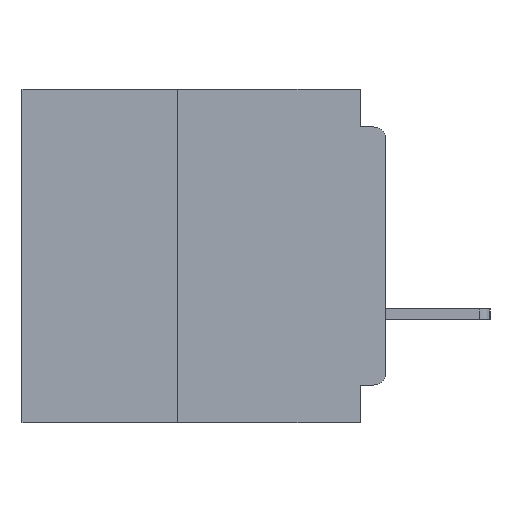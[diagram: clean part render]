
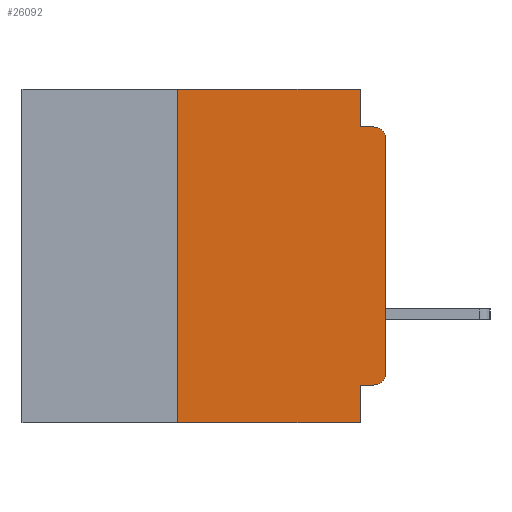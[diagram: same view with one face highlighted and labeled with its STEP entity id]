
A CAD part, left-side view. The second image highlights one B-rep face of the part: STEP entity #26092.
In plain terms, the highlighted planar face has unit normal (-1, 0, 0).
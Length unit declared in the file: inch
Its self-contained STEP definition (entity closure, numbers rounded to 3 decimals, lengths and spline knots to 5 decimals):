
#500 = CARTESIAN_POINT ( 'NONE',  ( 0., 0.437, 0. ) ) ;
#992 = VERTEX_POINT ( 'NONE', #31746 ) ;
#1232 = EDGE_CURVE ( 'NONE', #992, #51949, #61329, .T. ) ;
#2857 = CARTESIAN_POINT ( 'NONE',  ( 0., 0.031, 0. ) ) ;
#4072 = CARTESIAN_POINT ( 'NONE',  ( 0., 0.031, -0.045 ) ) ;
#5581 = VERTEX_POINT ( 'NONE', #11005 ) ;
#5593 = DIRECTION ( 'NONE',  ( 0., 0., 1. ) ) ;
#6571 = DIRECTION ( 'NONE',  ( 0., 1., 0. ) ) ;
#6765 = CARTESIAN_POINT ( 'NONE',  ( 0., 0., -0.045 ) ) ;
#6943 = AXIS2_PLACEMENT_3D ( 'NONE', #26610, #61513, #31609 ) ;
#7300 = VERTEX_POINT ( 'NONE', #53724 ) ;
#7449 = ORIENTED_EDGE ( 'NONE', *, *, #25702, .F. ) ;
#7754 = VECTOR ( 'NONE', #41854, 39.37008 ) ;
#8398 = ORIENTED_EDGE ( 'NONE', *, *, #21224, .F. ) ;
#8741 = CARTESIAN_POINT ( 'NONE',  ( 0., 0.031, -0.355 ) ) ;
#11005 = CARTESIAN_POINT ( 'NONE',  ( 0., 0.031, -0.4 ) ) ;
#11214 = CIRCLE ( 'NONE', #6943, 0.015 ) ;
#11303 = PLANE ( 'NONE',  #13007 ) ;
#11620 = VECTOR ( 'NONE', #24111, 39.37008 ) ;
#13007 = AXIS2_PLACEMENT_3D ( 'NONE', #41260, #16359, #51320 ) ;
#13833 = ORIENTED_EDGE ( 'NONE', *, *, #24499, .F. ) ;
#15007 = CARTESIAN_POINT ( 'NONE',  ( 0., 0.25, -0.4 ) ) ;
#15055 = VERTEX_POINT ( 'NONE', #15007 ) ;
#15559 = CARTESIAN_POINT ( 'NONE',  ( 0., 0.25, -0.4 ) ) ;
#15637 = ORIENTED_EDGE ( 'NONE', *, *, #37965, .F. ) ;
#16199 = VERTEX_POINT ( 'NONE', #8741 ) ;
#16359 = DIRECTION ( 'NONE',  ( 1., 0., 0. ) ) ;
#19058 = CARTESIAN_POINT ( 'NONE',  ( 0., 0.437, -0.4 ) ) ;
#19128 = VERTEX_POINT ( 'NONE', #58905 ) ;
#19398 = CARTESIAN_POINT ( 'NONE',  ( 0., 0.25, 0. ) ) ;
#19789 = ORIENTED_EDGE ( 'NONE', *, *, #22932, .T. ) ;
#20250 = LINE ( 'NONE', #20913, #33550 ) ;
#20913 = CARTESIAN_POINT ( 'NONE',  ( 0., 0., 0. ) ) ;
#20931 = VERTEX_POINT ( 'NONE', #19398 ) ;
#21178 = LINE ( 'NONE', #6765, #7754 ) ;
#21224 = EDGE_CURVE ( 'NONE', #41290, #51949, #21178, .T. ) ;
#22932 = EDGE_CURVE ( 'NONE', #7300, #992, #20250, .T. ) ;
#24111 = DIRECTION ( 'NONE',  ( 0., -1., 0. ) ) ;
#24387 = VECTOR ( 'NONE', #6571, 39.37008 ) ;
#24499 = EDGE_CURVE ( 'NONE', #16199, #5581, #54461, .T. ) ;
#24988 = LINE ( 'NONE', #19058, #11620 ) ;
#25702 = EDGE_CURVE ( 'NONE', #19128, #41290, #32363, .T. ) ;
#26092 = ADVANCED_FACE ( 'NONE', ( #60447 ), #11303, .F. ) ;
#26610 = CARTESIAN_POINT ( 'NONE',  ( 0., 0.015, -0.34 ) ) ;
#28370 = EDGE_CURVE ( 'NONE', #15055, #20931, #55471, .T. ) ;
#31390 = CARTESIAN_POINT ( 'NONE',  ( 0., 0.015, -0.355 ) ) ;
#31609 = DIRECTION ( 'NONE',  ( 0., 0., -1. ) ) ;
#31746 = CARTESIAN_POINT ( 'NONE',  ( 0., 0., -0.06 ) ) ;
#32363 = LINE ( 'NONE', #2857, #58949 ) ;
#33550 = VECTOR ( 'NONE', #50844, 39.37008 ) ;
#35780 = DIRECTION ( 'NONE',  ( 0., -1., 0. ) ) ;
#35940 = EDGE_LOOP ( 'NONE', ( #19789, #60717, #8398, #7449, #48199, #58741, #58434, #13833, #15637, #64451 ) ) ;
#36668 = EDGE_CURVE ( 'NONE', #51072, #7300, #11214, .T. ) ;
#37319 = DIRECTION ( 'NONE',  ( 0., 0., -1. ) ) ;
#37965 = EDGE_CURVE ( 'NONE', #51072, #16199, #49364, .T. ) ;
#38059 = DIRECTION ( 'NONE',  ( 0., 0., -1. ) ) ;
#41112 = VECTOR ( 'NONE', #37319, 39.37008 ) ;
#41260 = CARTESIAN_POINT ( 'NONE',  ( 0., 0.437, 0. ) ) ;
#41290 = VERTEX_POINT ( 'NONE', #4072 ) ;
#41667 = CARTESIAN_POINT ( 'NONE',  ( 0., 0., -0.355 ) ) ;
#41854 = DIRECTION ( 'NONE',  ( 0., -1., 0. ) ) ;
#42123 = CARTESIAN_POINT ( 'NONE',  ( 0., 0.031, -0.4 ) ) ;
#42150 = VECTOR ( 'NONE', #5593, 39.37008 ) ;
#42364 = CARTESIAN_POINT ( 'NONE',  ( 0., 0.015, -0.045 ) ) ;
#46923 = VECTOR ( 'NONE', #35780, 39.37008 ) ;
#47663 = EDGE_CURVE ( 'NONE', #20931, #19128, #61799, .T. ) ;
#48199 = ORIENTED_EDGE ( 'NONE', *, *, #47663, .F. ) ;
#49364 = LINE ( 'NONE', #41667, #24387 ) ;
#50844 = DIRECTION ( 'NONE',  ( 0., 0., 1. ) ) ;
#51072 = VERTEX_POINT ( 'NONE', #31390 ) ;
#51320 = DIRECTION ( 'NONE',  ( 0., 0., -1. ) ) ;
#51949 = VERTEX_POINT ( 'NONE', #42364 ) ;
#53167 = AXIS2_PLACEMENT_3D ( 'NONE', #63978, #55998, #56009 ) ;
#53724 = CARTESIAN_POINT ( 'NONE',  ( 0., 0., -0.34 ) ) ;
#54461 = LINE ( 'NONE', #42123, #41112 ) ;
#55471 = LINE ( 'NONE', #15559, #42150 ) ;
#55998 = DIRECTION ( 'NONE',  ( -1., 0., 0. ) ) ;
#56009 = DIRECTION ( 'NONE',  ( 0., 0., -1. ) ) ;
#57819 = EDGE_CURVE ( 'NONE', #15055, #5581, #24988, .T. ) ;
#58434 = ORIENTED_EDGE ( 'NONE', *, *, #57819, .T. ) ;
#58741 = ORIENTED_EDGE ( 'NONE', *, *, #28370, .F. ) ;
#58905 = CARTESIAN_POINT ( 'NONE',  ( 0., 0.031, 0. ) ) ;
#58949 = VECTOR ( 'NONE', #38059, 39.37008 ) ;
#60447 = FACE_OUTER_BOUND ( 'NONE', #35940, .T. ) ;
#60717 = ORIENTED_EDGE ( 'NONE', *, *, #1232, .T. ) ;
#61329 = CIRCLE ( 'NONE', #53167, 0.015 ) ;
#61513 = DIRECTION ( 'NONE',  ( -1., 0., 0. ) ) ;
#61799 = LINE ( 'NONE', #500, #46923 ) ;
#63978 = CARTESIAN_POINT ( 'NONE',  ( 0., 0.015, -0.06 ) ) ;
#64451 = ORIENTED_EDGE ( 'NONE', *, *, #36668, .T. ) ;
